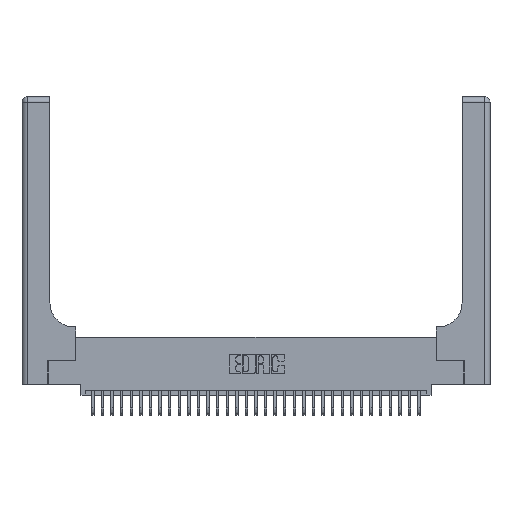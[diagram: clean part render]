
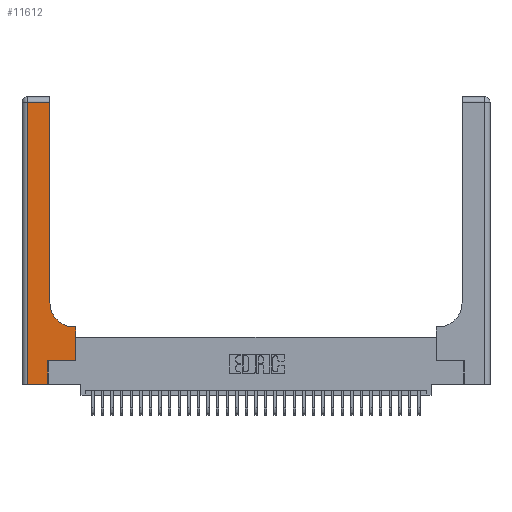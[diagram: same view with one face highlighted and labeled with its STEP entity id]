
A CAD part, top view. The second image highlights one B-rep face of the part: STEP entity #11612.
In plain terms, the highlighted planar face has unit normal (0, 0, 1).
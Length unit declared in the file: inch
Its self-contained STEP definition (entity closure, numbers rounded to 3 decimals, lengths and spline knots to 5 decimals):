
#42 = VERTEX_POINT ( 'NONE', #7275 ) ;
#196 = CARTESIAN_POINT ( 'NONE',  ( 0.2915, 2.94, 0.37 ) ) ;
#1060 = ORIENTED_EDGE ( 'NONE', *, *, #31613, .T. ) ;
#1201 = DIRECTION ( 'NONE',  ( 0., 1., 0. ) ) ;
#1483 = ORIENTED_EDGE ( 'NONE', *, *, #3403, .T. ) ;
#1691 = VERTEX_POINT ( 'NONE', #4470 ) ;
#1962 = ORIENTED_EDGE ( 'NONE', *, *, #2218, .T. ) ;
#2218 = EDGE_CURVE ( 'NONE', #10589, #8112, #27226, .T. ) ;
#3403 = EDGE_CURVE ( 'NONE', #26657, #30631, #4825, .T. ) ;
#3438 = LINE ( 'NONE', #32235, #29999 ) ;
#3505 = CARTESIAN_POINT ( 'NONE',  ( 0.2915, 0.6, 0.37 ) ) ;
#4369 = EDGE_CURVE ( 'NONE', #33007, #26657, #21826, .T. ) ;
#4470 = CARTESIAN_POINT ( 'NONE',  ( 0.06, 0., 0.37 ) ) ;
#4825 = LINE ( 'NONE', #17733, #33016 ) ;
#5710 = CARTESIAN_POINT ( 'NONE',  ( 0.2915, 3., 0.37 ) ) ;
#6298 = DIRECTION ( 'NONE',  ( -1., 0., 0. ) ) ;
#7275 = CARTESIAN_POINT ( 'NONE',  ( 0.5585, 0.6, 0.37 ) ) ;
#7692 = VERTEX_POINT ( 'NONE', #28275 ) ;
#7851 = CARTESIAN_POINT ( 'NONE',  ( 0., 0., 0.37 ) ) ;
#8112 = VERTEX_POINT ( 'NONE', #22208 ) ;
#10589 = VERTEX_POINT ( 'NONE', #11398 ) ;
#10628 = LINE ( 'NONE', #24262, #24421 ) ;
#11398 = CARTESIAN_POINT ( 'NONE',  ( 0.269, 0., 0.37 ) ) ;
#11612 = ADVANCED_FACE ( 'NONE', ( #17251 ), #28319, .F. ) ;
#13323 = EDGE_CURVE ( 'NONE', #7692, #33007, #18397, .T. ) ;
#14230 = CARTESIAN_POINT ( 'NONE',  ( 0.5585, 0.25, 0.37 ) ) ;
#14485 = VECTOR ( 'NONE', #30348, 39.37008 ) ;
#14699 = DIRECTION ( 'NONE',  ( -1., 0., 0. ) ) ;
#15311 = ORIENTED_EDGE ( 'NONE', *, *, #13323, .T. ) ;
#15318 = ORIENTED_EDGE ( 'NONE', *, *, #29031, .T. ) ;
#15682 = EDGE_LOOP ( 'NONE', ( #28468, #1483, #1060, #23481, #1962, #15318, #29421, #21334, #15311 ) ) ;
#16169 = CARTESIAN_POINT ( 'NONE',  ( 0.5415, 0.85, 0.37 ) ) ;
#16834 = VERTEX_POINT ( 'NONE', #14230 ) ;
#17251 = FACE_OUTER_BOUND ( 'NONE', #15682, .T. ) ;
#17509 = VECTOR ( 'NONE', #6298, 39.37008 ) ;
#17733 = CARTESIAN_POINT ( 'NONE',  ( 0., 2.94, 0.37 ) ) ;
#18397 = CIRCLE ( 'NONE', #29074, 0.25 ) ;
#18933 = DIRECTION ( 'NONE',  ( 1., 0., 0. ) ) ;
#19979 = VECTOR ( 'NONE', #1201, 39.37008 ) ;
#20126 = CARTESIAN_POINT ( 'NONE',  ( 0., 3., 0.37 ) ) ;
#20626 = EDGE_CURVE ( 'NONE', #16834, #42, #3438, .T. ) ;
#21334 = ORIENTED_EDGE ( 'NONE', *, *, #31466, .T. ) ;
#21826 = LINE ( 'NONE', #5710, #14485 ) ;
#22208 = CARTESIAN_POINT ( 'NONE',  ( 0.269, 0.25, 0.37 ) ) ;
#23054 = EDGE_CURVE ( 'NONE', #1691, #10589, #31515, .T. ) ;
#23481 = ORIENTED_EDGE ( 'NONE', *, *, #23054, .T. ) ;
#24130 = DIRECTION ( 'NONE',  ( 0., 1., 0. ) ) ;
#24262 = CARTESIAN_POINT ( 'NONE',  ( 0.269, 0.25, 0.37 ) ) ;
#24421 = VECTOR ( 'NONE', #26959, 39.37008 ) ;
#24458 = DIRECTION ( 'NONE',  ( 1., 0., 0. ) ) ;
#24741 = CARTESIAN_POINT ( 'NONE',  ( 0.06, 2.94, 0.37 ) ) ;
#25606 = LINE ( 'NONE', #3505, #17509 ) ;
#25698 = CARTESIAN_POINT ( 'NONE',  ( 0.269, 0., 0.37 ) ) ;
#26657 = VERTEX_POINT ( 'NONE', #196 ) ;
#26959 = DIRECTION ( 'NONE',  ( 1., 0., 0. ) ) ;
#27226 = LINE ( 'NONE', #25698, #19979 ) ;
#27684 = LINE ( 'NONE', #31378, #34010 ) ;
#28275 = CARTESIAN_POINT ( 'NONE',  ( 0.5415, 0.6, 0.37 ) ) ;
#28319 = PLANE ( 'NONE',  #30607 ) ;
#28468 = ORIENTED_EDGE ( 'NONE', *, *, #4369, .T. ) ;
#28652 = DIRECTION ( 'NONE',  ( -1., 0., 0. ) ) ;
#29031 = EDGE_CURVE ( 'NONE', #8112, #16834, #10628, .T. ) ;
#29074 = AXIS2_PLACEMENT_3D ( 'NONE', #16169, #35151, #18933 ) ;
#29421 = ORIENTED_EDGE ( 'NONE', *, *, #20626, .T. ) ;
#29999 = VECTOR ( 'NONE', #24130, 39.37008 ) ;
#30348 = DIRECTION ( 'NONE',  ( 0., 1., 0. ) ) ;
#30607 = AXIS2_PLACEMENT_3D ( 'NONE', #20126, #31024, #14699 ) ;
#30631 = VERTEX_POINT ( 'NONE', #24741 ) ;
#30641 = VECTOR ( 'NONE', #24458, 39.37008 ) ;
#31024 = DIRECTION ( 'NONE',  ( 0., 0., -1. ) ) ;
#31378 = CARTESIAN_POINT ( 'NONE',  ( 0.06, 3., 0.37 ) ) ;
#31466 = EDGE_CURVE ( 'NONE', #42, #7692, #25606, .T. ) ;
#31515 = LINE ( 'NONE', #7851, #30641 ) ;
#31613 = EDGE_CURVE ( 'NONE', #30631, #1691, #27684, .T. ) ;
#32235 = CARTESIAN_POINT ( 'NONE',  ( 0.5585, 0.25, 0.37 ) ) ;
#33007 = VERTEX_POINT ( 'NONE', #34845 ) ;
#33016 = VECTOR ( 'NONE', #28652, 39.37008 ) ;
#34010 = VECTOR ( 'NONE', #34086, 39.37008 ) ;
#34086 = DIRECTION ( 'NONE',  ( 0., -1., 0. ) ) ;
#34845 = CARTESIAN_POINT ( 'NONE',  ( 0.2915, 0.85, 0.37 ) ) ;
#35151 = DIRECTION ( 'NONE',  ( 0., 0., -1. ) ) ;
